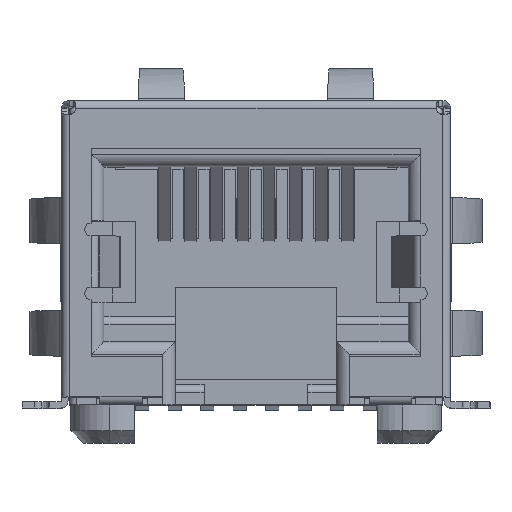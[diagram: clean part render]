
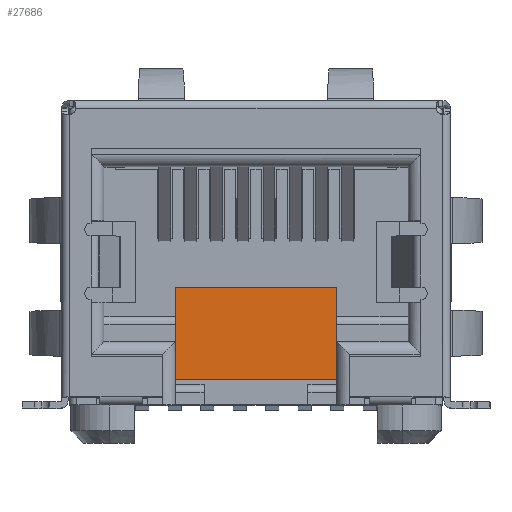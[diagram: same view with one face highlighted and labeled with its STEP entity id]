
A CAD part, top view. The second image highlights one B-rep face of the part: STEP entity #27686.
In plain terms, the highlighted planar face has unit normal (0, 0, 1).
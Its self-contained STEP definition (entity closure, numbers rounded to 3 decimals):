
#1453 = DIRECTION ( 'NONE',  ( -1., 0., 0. ) ) ;
#1560 = ORIENTED_EDGE ( 'NONE', *, *, #10026, .T. ) ;
#1801 = DIRECTION ( 'NONE',  ( 0., 1., 0. ) ) ;
#1819 = LINE ( 'NONE', #23379, #6268 ) ;
#1939 = VERTEX_POINT ( 'NONE', #24544 ) ;
#2724 = LINE ( 'NONE', #22231, #22121 ) ;
#3075 = VECTOR ( 'NONE', #18227, 1000. ) ;
#3872 = LINE ( 'NONE', #30973, #3075 ) ;
#5669 = EDGE_LOOP ( 'NONE', ( #26270, #1560, #30363, #10709 ) ) ;
#6268 = VECTOR ( 'NONE', #13197, 1000. ) ;
#8477 = EDGE_CURVE ( 'NONE', #24898, #32568, #17654, .T. ) ;
#10026 = EDGE_CURVE ( 'NONE', #13578, #32568, #2724, .T. ) ;
#10709 = ORIENTED_EDGE ( 'NONE', *, *, #11631, .F. ) ;
#11631 = EDGE_CURVE ( 'NONE', #1939, #24898, #3872, .T. ) ;
#12223 = EDGE_CURVE ( 'NONE', #13578, #1939, #1819, .T. ) ;
#13197 = DIRECTION ( 'NONE',  ( 0., -1., 0. ) ) ;
#13543 = FACE_OUTER_BOUND ( 'NONE', #5669, .T. ) ;
#13578 = VERTEX_POINT ( 'NONE', #20452 ) ;
#15941 = PLANE ( 'NONE',  #30218 ) ;
#16044 = CARTESIAN_POINT ( 'NONE',  ( -3.15, 1., -4.7 ) ) ;
#17654 = LINE ( 'NONE', #22013, #18865 ) ;
#18227 = DIRECTION ( 'NONE',  ( -1., 0., 0. ) ) ;
#18552 = CARTESIAN_POINT ( 'NONE',  ( -3.276, 4.672, -4.7 ) ) ;
#18865 = VECTOR ( 'NONE', #1801, 1000. ) ;
#20452 = CARTESIAN_POINT ( 'NONE',  ( 3.15, 4.6, -4.7 ) ) ;
#21279 = DIRECTION ( 'NONE',  ( 1., 0., 0. ) ) ;
#22013 = CARTESIAN_POINT ( 'NONE',  ( -3.15, 2.8, -4.7 ) ) ;
#22121 = VECTOR ( 'NONE', #1453, 1000. ) ;
#22231 = CARTESIAN_POINT ( 'NONE',  ( 0., 4.6, -4.7 ) ) ;
#22835 = CARTESIAN_POINT ( 'NONE',  ( -3.15, 4.6, -4.7 ) ) ;
#23379 = CARTESIAN_POINT ( 'NONE',  ( 3.15, 2.8, -4.7 ) ) ;
#23636 = DIRECTION ( 'NONE',  ( 0., 0., -1. ) ) ;
#24544 = CARTESIAN_POINT ( 'NONE',  ( 3.15, 1., -4.7 ) ) ;
#24898 = VERTEX_POINT ( 'NONE', #16044 ) ;
#26270 = ORIENTED_EDGE ( 'NONE', *, *, #12223, .F. ) ;
#27686 = ADVANCED_FACE ( 'NONE', ( #13543 ), #15941, .F. ) ;
#30218 = AXIS2_PLACEMENT_3D ( 'NONE', #18552, #23636, #21279 ) ;
#30363 = ORIENTED_EDGE ( 'NONE', *, *, #8477, .F. ) ;
#30973 = CARTESIAN_POINT ( 'NONE',  ( 0., 1., -4.7 ) ) ;
#32568 = VERTEX_POINT ( 'NONE', #22835 ) ;
